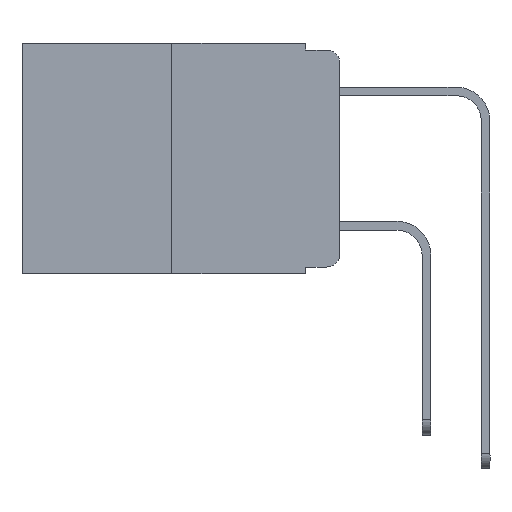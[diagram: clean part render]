
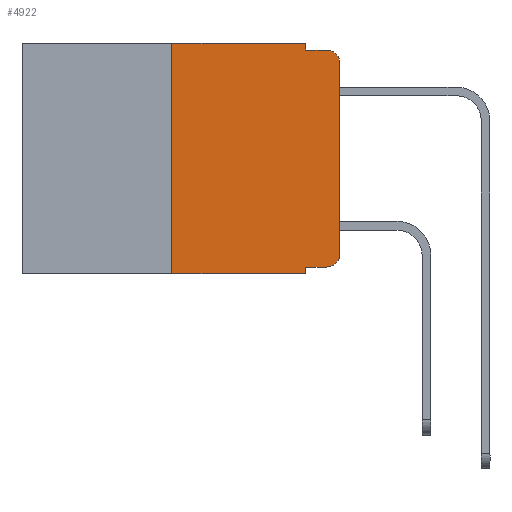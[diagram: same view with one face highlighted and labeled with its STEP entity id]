
A CAD part, left-side view. The second image highlights one B-rep face of the part: STEP entity #4922.
In plain terms, the highlighted planar face has unit normal (-1, 0, 0).
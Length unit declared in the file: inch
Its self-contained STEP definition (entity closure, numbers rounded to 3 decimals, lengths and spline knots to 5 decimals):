
#3 = CIRCLE ( 'NONE', #7485, 0.02 ) ;
#36 = CARTESIAN_POINT ( 'NONE',  ( 0., 0.25, -0.343 ) ) ;
#83 = VECTOR ( 'NONE', #11064, 39.37008 ) ;
#254 = EDGE_LOOP ( 'NONE', ( #3711, #7794, #3067, #4527, #11916, #6341, #6675, #2876, #6172, #8171 ) ) ;
#667 = DIRECTION ( 'NONE',  ( 0., -1., 0. ) ) ;
#745 = VECTOR ( 'NONE', #3224, 39.37008 ) ;
#1051 = VERTEX_POINT ( 'NONE', #10218 ) ;
#1213 = VECTOR ( 'NONE', #6253, 39.37008 ) ;
#1318 = CARTESIAN_POINT ( 'NONE',  ( 0., 0.02, -0.03 ) ) ;
#1514 = CARTESIAN_POINT ( 'NONE',  ( 0., 0., -0.313 ) ) ;
#1544 = CARTESIAN_POINT ( 'NONE',  ( 0., 0.051, 0. ) ) ;
#1613 = DIRECTION ( 'NONE',  ( 0., 0., -1. ) ) ;
#2005 = VERTEX_POINT ( 'NONE', #11618 ) ;
#2067 = EDGE_CURVE ( 'NONE', #11627, #2192, #10686, .T. ) ;
#2192 = VERTEX_POINT ( 'NONE', #3031 ) ;
#2438 = CARTESIAN_POINT ( 'NONE',  ( 0., 0.051, -0.333 ) ) ;
#2532 = EDGE_CURVE ( 'NONE', #5161, #1051, #2952, .T. ) ;
#2552 = DIRECTION ( 'NONE',  ( -1., 0., 0. ) ) ;
#2704 = DIRECTION ( 'NONE',  ( 0., 0., -1. ) ) ;
#2876 = ORIENTED_EDGE ( 'NONE', *, *, #8001, .F. ) ;
#2952 = LINE ( 'NONE', #5881, #83 ) ;
#3031 = CARTESIAN_POINT ( 'NONE',  ( 0., 0.051, -0.01 ) ) ;
#3067 = ORIENTED_EDGE ( 'NONE', *, *, #12914, .F. ) ;
#3189 = LINE ( 'NONE', #9125, #7547 ) ;
#3224 = DIRECTION ( 'NONE',  ( 0., -1., 0. ) ) ;
#3354 = EDGE_CURVE ( 'NONE', #2005, #5161, #3, .T. ) ;
#3419 = DIRECTION ( 'NONE',  ( 0., 0., -1. ) ) ;
#3656 = VERTEX_POINT ( 'NONE', #12337 ) ;
#3711 = ORIENTED_EDGE ( 'NONE', *, *, #2532, .T. ) ;
#3756 = CARTESIAN_POINT ( 'NONE',  ( 0., 0.25, 0. ) ) ;
#4352 = CARTESIAN_POINT ( 'NONE',  ( 0., 0.02, -0.313 ) ) ;
#4466 = DIRECTION ( 'NONE',  ( 0., 0., -1. ) ) ;
#4527 = ORIENTED_EDGE ( 'NONE', *, *, #2067, .F. ) ;
#4533 = CARTESIAN_POINT ( 'NONE',  ( 0., 0.051, -0.333 ) ) ;
#4786 = CARTESIAN_POINT ( 'NONE',  ( 0., 0.051, -0.343 ) ) ;
#4833 = DIRECTION ( 'NONE',  ( 1., 0., 0. ) ) ;
#4922 = ADVANCED_FACE ( 'NONE', ( #11750 ), #5827, .F. ) ;
#5082 = LINE ( 'NONE', #10010, #9520 ) ;
#5120 = DIRECTION ( 'NONE',  ( 0., 0., -1. ) ) ;
#5161 = VERTEX_POINT ( 'NONE', #1514 ) ;
#5196 = VERTEX_POINT ( 'NONE', #4533 ) ;
#5379 = DIRECTION ( 'NONE',  ( 0., -1., 0. ) ) ;
#5827 = PLANE ( 'NONE',  #9724 ) ;
#5881 = CARTESIAN_POINT ( 'NONE',  ( 0., 0., 0. ) ) ;
#5964 = CARTESIAN_POINT ( 'NONE',  ( 0., 0.473, -0.343 ) ) ;
#6125 = EDGE_CURVE ( 'NONE', #5196, #2005, #9506, .T. ) ;
#6172 = ORIENTED_EDGE ( 'NONE', *, *, #6125, .T. ) ;
#6253 = DIRECTION ( 'NONE',  ( 0., -1., 0. ) ) ;
#6341 = ORIENTED_EDGE ( 'NONE', *, *, #10641, .F. ) ;
#6675 = ORIENTED_EDGE ( 'NONE', *, *, #10251, .T. ) ;
#6721 = AXIS2_PLACEMENT_3D ( 'NONE', #1318, #9403, #4466 ) ;
#7485 = AXIS2_PLACEMENT_3D ( 'NONE', #4352, #2552, #3419 ) ;
#7543 = EDGE_CURVE ( 'NONE', #10028, #11627, #11893, .T. ) ;
#7547 = VECTOR ( 'NONE', #5120, 39.37008 ) ;
#7794 = ORIENTED_EDGE ( 'NONE', *, *, #9467, .T. ) ;
#8001 = EDGE_CURVE ( 'NONE', #5196, #12724, #3189, .T. ) ;
#8171 = ORIENTED_EDGE ( 'NONE', *, *, #3354, .T. ) ;
#8245 = CARTESIAN_POINT ( 'NONE',  ( 0., 0.051, 0. ) ) ;
#8381 = CARTESIAN_POINT ( 'NONE',  ( 0., 0.051, -0.01 ) ) ;
#9125 = CARTESIAN_POINT ( 'NONE',  ( 0., 0.051, 0. ) ) ;
#9183 = LINE ( 'NONE', #8381, #1213 ) ;
#9403 = DIRECTION ( 'NONE',  ( -1., 0., 0. ) ) ;
#9467 = EDGE_CURVE ( 'NONE', #1051, #3656, #10532, .T. ) ;
#9506 = LINE ( 'NONE', #2438, #12171 ) ;
#9520 = VECTOR ( 'NONE', #12197, 39.37008 ) ;
#9654 = VECTOR ( 'NONE', #667, 39.37008 ) ;
#9724 = AXIS2_PLACEMENT_3D ( 'NONE', #11817, #4833, #1613 ) ;
#10010 = CARTESIAN_POINT ( 'NONE',  ( 0., 0.25, 0. ) ) ;
#10028 = VERTEX_POINT ( 'NONE', #3756 ) ;
#10218 = CARTESIAN_POINT ( 'NONE',  ( 0., 0., -0.03 ) ) ;
#10251 = EDGE_CURVE ( 'NONE', #12532, #12724, #12287, .T. ) ;
#10532 = CIRCLE ( 'NONE', #6721, 0.02 ) ;
#10641 = EDGE_CURVE ( 'NONE', #12532, #10028, #5082, .T. ) ;
#10686 = LINE ( 'NONE', #1544, #11966 ) ;
#11064 = DIRECTION ( 'NONE',  ( 0., 0., 1. ) ) ;
#11618 = CARTESIAN_POINT ( 'NONE',  ( 0., 0.02, -0.333 ) ) ;
#11627 = VERTEX_POINT ( 'NONE', #8245 ) ;
#11750 = FACE_OUTER_BOUND ( 'NONE', #254, .T. ) ;
#11817 = CARTESIAN_POINT ( 'NONE',  ( 0., 0.473, 0. ) ) ;
#11893 = LINE ( 'NONE', #12764, #9654 ) ;
#11916 = ORIENTED_EDGE ( 'NONE', *, *, #7543, .F. ) ;
#11966 = VECTOR ( 'NONE', #2704, 39.37008 ) ;
#12171 = VECTOR ( 'NONE', #5379, 39.37008 ) ;
#12197 = DIRECTION ( 'NONE',  ( 0., 0., 1. ) ) ;
#12287 = LINE ( 'NONE', #5964, #745 ) ;
#12337 = CARTESIAN_POINT ( 'NONE',  ( 0., 0.02, -0.01 ) ) ;
#12532 = VERTEX_POINT ( 'NONE', #36 ) ;
#12724 = VERTEX_POINT ( 'NONE', #4786 ) ;
#12764 = CARTESIAN_POINT ( 'NONE',  ( 0., 0.473, 0. ) ) ;
#12914 = EDGE_CURVE ( 'NONE', #2192, #3656, #9183, .T. ) ;
